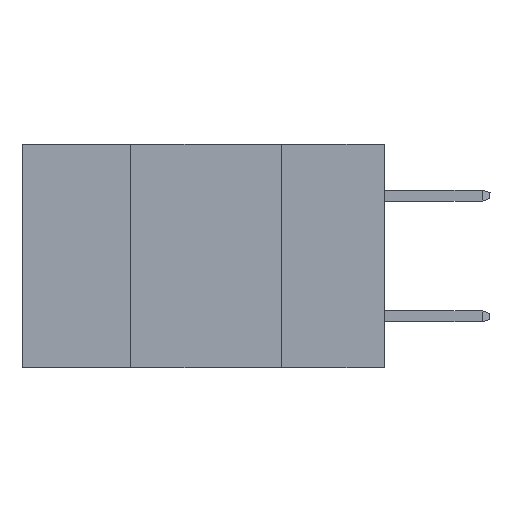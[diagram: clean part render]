
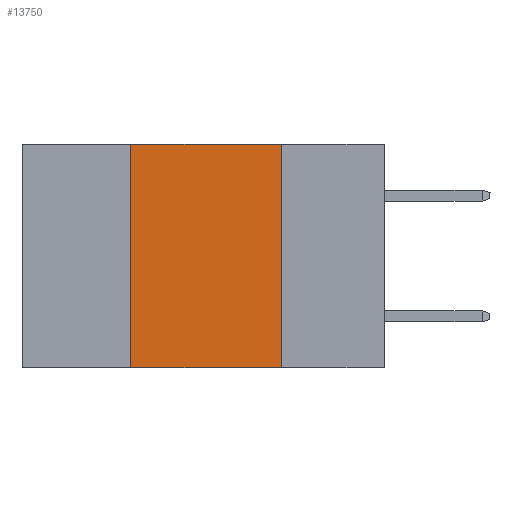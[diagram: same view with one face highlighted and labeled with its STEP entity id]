
A CAD part, left-side view. The second image highlights one B-rep face of the part: STEP entity #13750.
In plain terms, the highlighted planar face has unit normal (-1, 0, 0).
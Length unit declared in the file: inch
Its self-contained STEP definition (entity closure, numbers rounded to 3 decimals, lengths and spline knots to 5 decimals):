
#853 = DIRECTION ( 'NONE',  ( 0., -1., 0. ) ) ;
#2092 = CARTESIAN_POINT ( 'NONE',  ( 0., 0.42, 0. ) ) ;
#2194 = EDGE_LOOP ( 'NONE', ( #11893, #11362, #8002, #7493 ) ) ;
#4579 = EDGE_CURVE ( 'NONE', #19407, #9654, #23542, .T. ) ;
#5518 = VECTOR ( 'NONE', #23033, 39.37008 ) ;
#6475 = CARTESIAN_POINT ( 'NONE',  ( 0., 0.6, 0. ) ) ;
#7389 = VERTEX_POINT ( 'NONE', #16901 ) ;
#7493 = ORIENTED_EDGE ( 'NONE', *, *, #15933, .T. ) ;
#7831 = DIRECTION ( 'NONE',  ( 0., -1., 0. ) ) ;
#8002 = ORIENTED_EDGE ( 'NONE', *, *, #17183, .F. ) ;
#9654 = VERTEX_POINT ( 'NONE', #14672 ) ;
#9754 = FACE_OUTER_BOUND ( 'NONE', #2194, .T. ) ;
#10913 = VECTOR ( 'NONE', #853, 39.37008 ) ;
#11362 = ORIENTED_EDGE ( 'NONE', *, *, #4579, .F. ) ;
#11673 = CARTESIAN_POINT ( 'NONE',  ( 0., 0.17, 0. ) ) ;
#11707 = CARTESIAN_POINT ( 'NONE',  ( 0., 0.42, 0. ) ) ;
#11893 = ORIENTED_EDGE ( 'NONE', *, *, #24058, .F. ) ;
#12242 = DIRECTION ( 'NONE',  ( 0., 0., -1. ) ) ;
#12379 = LINE ( 'NONE', #11673, #13274 ) ;
#12966 = AXIS2_PLACEMENT_3D ( 'NONE', #18172, #23750, #20061 ) ;
#12992 = VECTOR ( 'NONE', #7831, 39.37008 ) ;
#13274 = VECTOR ( 'NONE', #12242, 39.37008 ) ;
#13750 = ADVANCED_FACE ( 'NONE', ( #9754 ), #14509, .F. ) ;
#14509 = PLANE ( 'NONE',  #12966 ) ;
#14672 = CARTESIAN_POINT ( 'NONE',  ( 0., 0.17, 0. ) ) ;
#15933 = EDGE_CURVE ( 'NONE', #7389, #21363, #18846, .T. ) ;
#16901 = CARTESIAN_POINT ( 'NONE',  ( 0., 0.42, -0.37 ) ) ;
#17183 = EDGE_CURVE ( 'NONE', #7389, #19407, #19088, .T. ) ;
#17476 = CARTESIAN_POINT ( 'NONE',  ( 0., 0.6, -0.37 ) ) ;
#18172 = CARTESIAN_POINT ( 'NONE',  ( 0., 0.6, 0. ) ) ;
#18846 = LINE ( 'NONE', #17476, #12992 ) ;
#19088 = LINE ( 'NONE', #11707, #5518 ) ;
#19407 = VERTEX_POINT ( 'NONE', #2092 ) ;
#20061 = DIRECTION ( 'NONE',  ( 0., 0., -1. ) ) ;
#20972 = CARTESIAN_POINT ( 'NONE',  ( 0., 0.17, -0.37 ) ) ;
#21363 = VERTEX_POINT ( 'NONE', #20972 ) ;
#23033 = DIRECTION ( 'NONE',  ( 0., 0., 1. ) ) ;
#23542 = LINE ( 'NONE', #6475, #10913 ) ;
#23750 = DIRECTION ( 'NONE',  ( 1., 0., 0. ) ) ;
#24058 = EDGE_CURVE ( 'NONE', #9654, #21363, #12379, .T. ) ;
